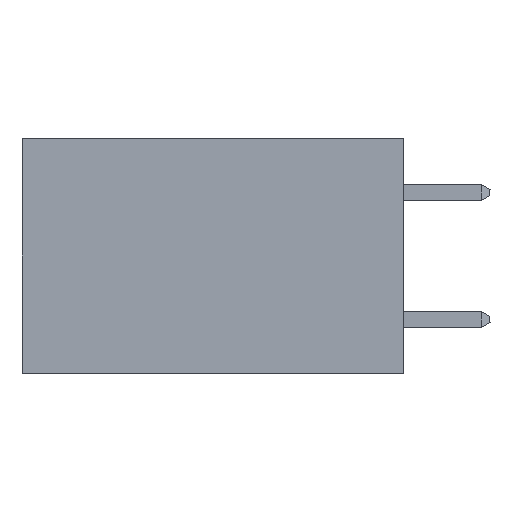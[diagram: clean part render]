
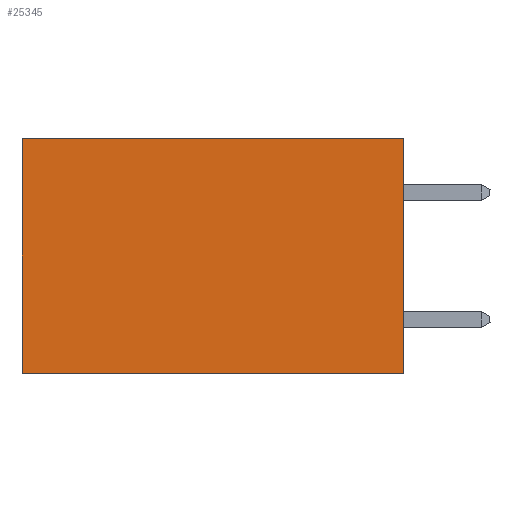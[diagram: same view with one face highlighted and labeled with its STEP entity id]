
A CAD part, left-side view. The second image highlights one B-rep face of the part: STEP entity #25345.
In plain terms, the highlighted planar face has unit normal (-1, 0, 0).
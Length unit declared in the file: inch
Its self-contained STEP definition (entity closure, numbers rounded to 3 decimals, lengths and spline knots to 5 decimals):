
#195 = VECTOR ( 'NONE', #28304, 39.37008 ) ;
#1996 = ORIENTED_EDGE ( 'NONE', *, *, #11130, .F. ) ;
#2903 = EDGE_CURVE ( 'NONE', #29937, #21891, #13830, .T. ) ;
#2962 = VECTOR ( 'NONE', #13873, 39.37008 ) ;
#5583 = ORIENTED_EDGE ( 'NONE', *, *, #2903, .F. ) ;
#5709 = VERTEX_POINT ( 'NONE', #13886 ) ;
#5893 = DIRECTION ( 'NONE',  ( 0., 1., 0. ) ) ;
#6325 = VERTEX_POINT ( 'NONE', #11885 ) ;
#7863 = ORIENTED_EDGE ( 'NONE', *, *, #29360, .T. ) ;
#8194 = DIRECTION ( 'NONE',  ( 1., 0., 0. ) ) ;
#9369 = CARTESIAN_POINT ( 'NONE',  ( 0.2875, 0., 0. ) ) ;
#11130 = EDGE_CURVE ( 'NONE', #21891, #6325, #20453, .T. ) ;
#11289 = CARTESIAN_POINT ( 'NONE',  ( 0.2875, 0., 0. ) ) ;
#11348 = CARTESIAN_POINT ( 'NONE',  ( 0.2875, 0., 0. ) ) ;
#11822 = DIRECTION ( 'NONE',  ( 0., 1., 0. ) ) ;
#11885 = CARTESIAN_POINT ( 'NONE',  ( 0.2875, 0.6, -0.37 ) ) ;
#12663 = DIRECTION ( 'NONE',  ( 0., 0., -1. ) ) ;
#13830 = LINE ( 'NONE', #11289, #195 ) ;
#13873 = DIRECTION ( 'NONE',  ( 0., 0., -1. ) ) ;
#13886 = CARTESIAN_POINT ( 'NONE',  ( 0.2875, 0.6, 0. ) ) ;
#14017 = LINE ( 'NONE', #9369, #28508 ) ;
#15926 = FACE_OUTER_BOUND ( 'NONE', #25318, .T. ) ;
#17508 = AXIS2_PLACEMENT_3D ( 'NONE', #24863, #8194, #12663 ) ;
#20453 = LINE ( 'NONE', #22684, #23504 ) ;
#21891 = VERTEX_POINT ( 'NONE', #24939 ) ;
#22684 = CARTESIAN_POINT ( 'NONE',  ( 0.2875, 0., -0.37 ) ) ;
#23504 = VECTOR ( 'NONE', #5893, 39.37008 ) ;
#24863 = CARTESIAN_POINT ( 'NONE',  ( 0.2875, 0., 0. ) ) ;
#24939 = CARTESIAN_POINT ( 'NONE',  ( 0.2875, 0., -0.37 ) ) ;
#25318 = EDGE_LOOP ( 'NONE', ( #25713, #1996, #5583, #7863 ) ) ;
#25345 = ADVANCED_FACE ( 'NONE', ( #15926 ), #27642, .F. ) ;
#25713 = ORIENTED_EDGE ( 'NONE', *, *, #29983, .T. ) ;
#26229 = CARTESIAN_POINT ( 'NONE',  ( 0.2875, 0.6, 0. ) ) ;
#27642 = PLANE ( 'NONE',  #17508 ) ;
#28304 = DIRECTION ( 'NONE',  ( 0., 0., -1. ) ) ;
#28508 = VECTOR ( 'NONE', #11822, 39.37008 ) ;
#29360 = EDGE_CURVE ( 'NONE', #29937, #5709, #14017, .T. ) ;
#29930 = LINE ( 'NONE', #26229, #2962 ) ;
#29937 = VERTEX_POINT ( 'NONE', #11348 ) ;
#29983 = EDGE_CURVE ( 'NONE', #5709, #6325, #29930, .T. ) ;
